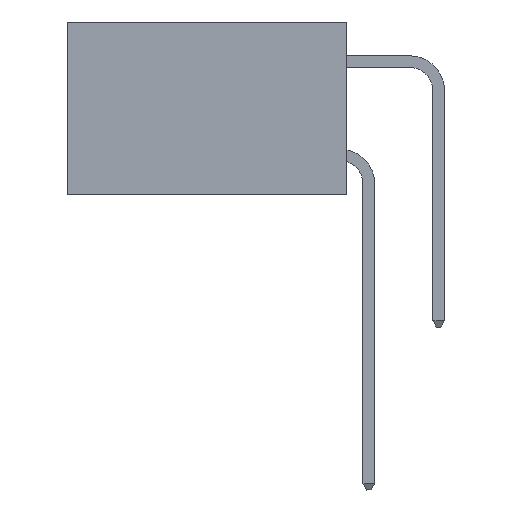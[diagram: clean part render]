
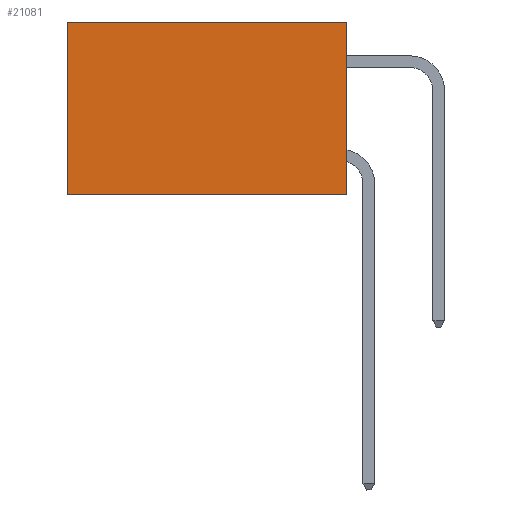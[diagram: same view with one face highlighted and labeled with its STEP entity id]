
A CAD part, left-side view. The second image highlights one B-rep face of the part: STEP entity #21081.
In plain terms, the highlighted planar face has unit normal (-1, 0, 0).
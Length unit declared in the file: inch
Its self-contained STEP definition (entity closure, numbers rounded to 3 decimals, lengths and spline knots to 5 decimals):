
#678 = VECTOR ( 'NONE', #19138, 39.37008 ) ;
#873 = ORIENTED_EDGE ( 'NONE', *, *, #3935, .F. ) ;
#1054 = CARTESIAN_POINT ( 'NONE',  ( 0.2875, 0.6, 0. ) ) ;
#1195 = EDGE_CURVE ( 'NONE', #17750, #11300, #14020, .T. ) ;
#2085 = ORIENTED_EDGE ( 'NONE', *, *, #1195, .F. ) ;
#3316 = CARTESIAN_POINT ( 'NONE',  ( 0.2875, 0., 0. ) ) ;
#3722 = AXIS2_PLACEMENT_3D ( 'NONE', #11375, #15524, #5568 ) ;
#3935 = EDGE_CURVE ( 'NONE', #11300, #4972, #17282, .T. ) ;
#4972 = VERTEX_POINT ( 'NONE', #21754 ) ;
#5072 = VERTEX_POINT ( 'NONE', #23375 ) ;
#5087 = DIRECTION ( 'NONE',  ( 0., 1., 0. ) ) ;
#5568 = DIRECTION ( 'NONE',  ( 0., 0., -1. ) ) ;
#6485 = EDGE_CURVE ( 'NONE', #17750, #5072, #10767, .T. ) ;
#7937 = CARTESIAN_POINT ( 'NONE',  ( 0.2875, 0., -0.37 ) ) ;
#9541 = VECTOR ( 'NONE', #5087, 39.37008 ) ;
#10767 = LINE ( 'NONE', #16770, #9541 ) ;
#11087 = FACE_OUTER_BOUND ( 'NONE', #18366, .T. ) ;
#11300 = VERTEX_POINT ( 'NONE', #19864 ) ;
#11375 = CARTESIAN_POINT ( 'NONE',  ( 0.2875, 0., 0. ) ) ;
#11863 = DIRECTION ( 'NONE',  ( 0., 1., 0. ) ) ;
#12285 = LINE ( 'NONE', #1054, #678 ) ;
#13614 = VECTOR ( 'NONE', #11863, 39.37008 ) ;
#13663 = EDGE_CURVE ( 'NONE', #5072, #4972, #12285, .T. ) ;
#14020 = LINE ( 'NONE', #16999, #20432 ) ;
#15524 = DIRECTION ( 'NONE',  ( 1., 0., 0. ) ) ;
#16770 = CARTESIAN_POINT ( 'NONE',  ( 0.2875, 0., 0. ) ) ;
#16999 = CARTESIAN_POINT ( 'NONE',  ( 0.2875, 0., 0. ) ) ;
#17282 = LINE ( 'NONE', #7937, #13614 ) ;
#17750 = VERTEX_POINT ( 'NONE', #3316 ) ;
#18366 = EDGE_LOOP ( 'NONE', ( #19507, #873, #2085, #22684 ) ) ;
#19116 = PLANE ( 'NONE',  #3722 ) ;
#19138 = DIRECTION ( 'NONE',  ( 0., 0., -1. ) ) ;
#19507 = ORIENTED_EDGE ( 'NONE', *, *, #13663, .T. ) ;
#19864 = CARTESIAN_POINT ( 'NONE',  ( 0.2875, 0., -0.37 ) ) ;
#20432 = VECTOR ( 'NONE', #21243, 39.37008 ) ;
#21081 = ADVANCED_FACE ( 'NONE', ( #11087 ), #19116, .F. ) ;
#21243 = DIRECTION ( 'NONE',  ( 0., 0., -1. ) ) ;
#21754 = CARTESIAN_POINT ( 'NONE',  ( 0.2875, 0.6, -0.37 ) ) ;
#22684 = ORIENTED_EDGE ( 'NONE', *, *, #6485, .T. ) ;
#23375 = CARTESIAN_POINT ( 'NONE',  ( 0.2875, 0.6, 0. ) ) ;
